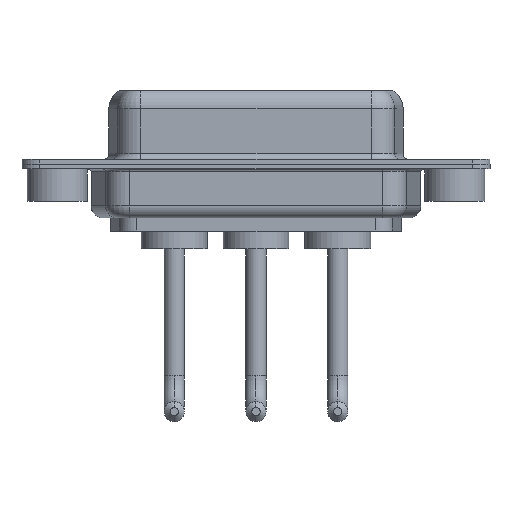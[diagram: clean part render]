
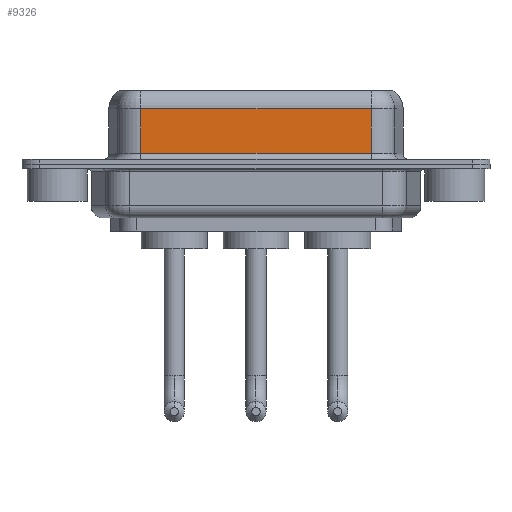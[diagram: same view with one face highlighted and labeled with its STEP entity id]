
A CAD part, front view. The second image highlights one B-rep face of the part: STEP entity #9326.
In plain terms, the highlighted planar face has unit normal (0, -1, 0).
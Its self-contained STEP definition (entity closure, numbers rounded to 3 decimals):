
#419 = DIRECTION ( 'NONE',  ( 0., 0., -1. ) ) ;
#805 = LINE ( 'NONE', #4467, #9854 ) ;
#922 = VERTEX_POINT ( 'NONE', #4525 ) ;
#1012 = EDGE_LOOP ( 'NONE', ( #11981, #1584, #7982, #5784 ) ) ;
#1584 = ORIENTED_EDGE ( 'NONE', *, *, #11011, .T. ) ;
#3373 = CARTESIAN_POINT ( 'NONE',  ( 26.287, -3.95, 4.65 ) ) ;
#4226 = PLANE ( 'NONE',  #7639 ) ;
#4403 = DIRECTION ( 'NONE',  ( 1., 0., 0. ) ) ;
#4467 = CARTESIAN_POINT ( 'NONE',  ( 26.287, -3.95, 0.9 ) ) ;
#4525 = CARTESIAN_POINT ( 'NONE',  ( 7.013, -3.95, 0.9 ) ) ;
#5095 = FACE_OUTER_BOUND ( 'NONE', #1012, .T. ) ;
#5125 = VECTOR ( 'NONE', #11268, 1000. ) ;
#5706 = CARTESIAN_POINT ( 'NONE',  ( 26.287, -3.95, 6.4 ) ) ;
#5784 = ORIENTED_EDGE ( 'NONE', *, *, #9429, .T. ) ;
#5828 = CARTESIAN_POINT ( 'NONE',  ( 26.287, -3.95, 4.65 ) ) ;
#6880 = CARTESIAN_POINT ( 'NONE',  ( 7.013, -3.95, 6.4 ) ) ;
#7639 = AXIS2_PLACEMENT_3D ( 'NONE', #9764, #10827, #8066 ) ;
#7683 = DIRECTION ( 'NONE',  ( 0., 0., -1. ) ) ;
#7982 = ORIENTED_EDGE ( 'NONE', *, *, #8007, .T. ) ;
#8007 = EDGE_CURVE ( 'NONE', #8822, #922, #11819, .T. ) ;
#8066 = DIRECTION ( 'NONE',  ( 0., 0., 1. ) ) ;
#8514 = LINE ( 'NONE', #5706, #12020 ) ;
#8540 = VERTEX_POINT ( 'NONE', #11232 ) ;
#8802 = VERTEX_POINT ( 'NONE', #3373 ) ;
#8822 = VERTEX_POINT ( 'NONE', #10966 ) ;
#9210 = VECTOR ( 'NONE', #419, 1000. ) ;
#9326 = ADVANCED_FACE ( 'NONE', ( #5095 ), #4226, .F. ) ;
#9429 = EDGE_CURVE ( 'NONE', #922, #8540, #805, .T. ) ;
#9764 = CARTESIAN_POINT ( 'NONE',  ( 26.287, -3.95, 6.4 ) ) ;
#9771 = EDGE_CURVE ( 'NONE', #8802, #8540, #8514, .T. ) ;
#9854 = VECTOR ( 'NONE', #4403, 1000. ) ;
#10573 = LINE ( 'NONE', #5828, #5125 ) ;
#10827 = DIRECTION ( 'NONE',  ( 0., 1., 0. ) ) ;
#10966 = CARTESIAN_POINT ( 'NONE',  ( 7.013, -3.95, 4.65 ) ) ;
#11011 = EDGE_CURVE ( 'NONE', #8802, #8822, #10573, .T. ) ;
#11232 = CARTESIAN_POINT ( 'NONE',  ( 26.287, -3.95, 0.9 ) ) ;
#11268 = DIRECTION ( 'NONE',  ( -1., 0., 0. ) ) ;
#11819 = LINE ( 'NONE', #6880, #9210 ) ;
#11981 = ORIENTED_EDGE ( 'NONE', *, *, #9771, .F. ) ;
#12020 = VECTOR ( 'NONE', #7683, 1000. ) ;
